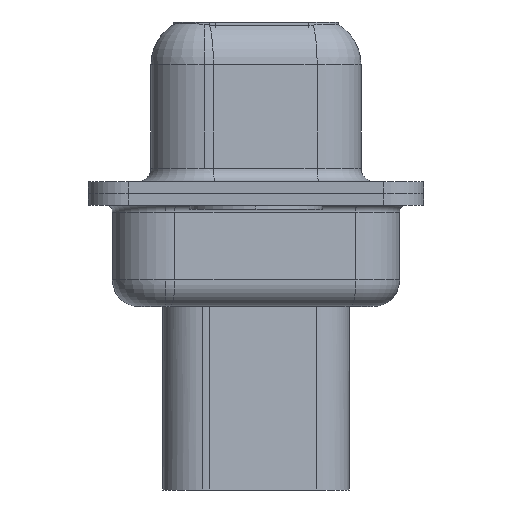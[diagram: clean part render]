
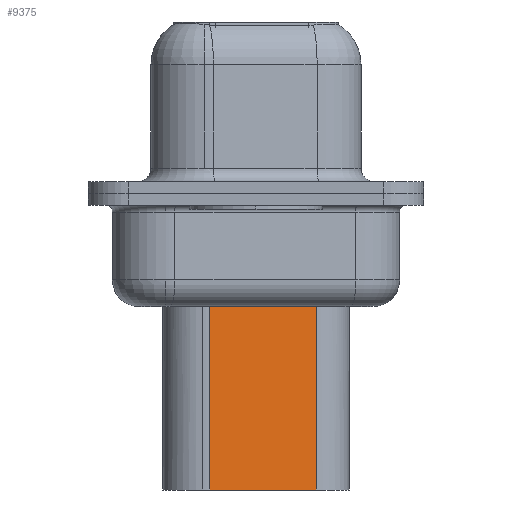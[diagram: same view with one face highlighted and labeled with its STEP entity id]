
A CAD part, left-side view. The second image highlights one B-rep face of the part: STEP entity #9375.
In plain terms, the highlighted planar face has unit normal (-0.985, -0.174, 0).
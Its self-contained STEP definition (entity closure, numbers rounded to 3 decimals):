
#28 = VECTOR ( 'NONE', #10240, 1000. ) ;
#296 = DIRECTION ( 'NONE',  ( -0.174, 0.985, 0. ) ) ;
#1216 = LINE ( 'NONE', #3573, #3936 ) ;
#1511 = EDGE_CURVE ( 'NONE', #6436, #9816, #1216, .T. ) ;
#1523 = EDGE_LOOP ( 'NONE', ( #1975, #10669, #6232, #9168 ) ) ;
#1604 = CARTESIAN_POINT ( 'NONE',  ( 4.524, 1.74, -3.975 ) ) ;
#1975 = ORIENTED_EDGE ( 'NONE', *, *, #5110, .F. ) ;
#2356 = EDGE_CURVE ( 'NONE', #5123, #9816, #5255, .T. ) ;
#3018 = PLANE ( 'NONE',  #7346 ) ;
#3091 = CARTESIAN_POINT ( 'NONE',  ( 5.229, -2.26, -3.975 ) ) ;
#3573 = CARTESIAN_POINT ( 'NONE',  ( 4.524, 1.74, -3.1 ) ) ;
#3772 = CARTESIAN_POINT ( 'NONE',  ( 4.524, 1.74, -3.1 ) ) ;
#3780 = DIRECTION ( 'NONE',  ( 0., 0., -1. ) ) ;
#3936 = VECTOR ( 'NONE', #3780, 1000. ) ;
#3957 = VERTEX_POINT ( 'NONE', #3091 ) ;
#4411 = LINE ( 'NONE', #9379, #4793 ) ;
#4793 = VECTOR ( 'NONE', #10362, 1000. ) ;
#5110 = EDGE_CURVE ( 'NONE', #3957, #5123, #4411, .T. ) ;
#5123 = VERTEX_POINT ( 'NONE', #8883 ) ;
#5255 = LINE ( 'NONE', #5914, #7487 ) ;
#5568 = FACE_OUTER_BOUND ( 'NONE', #1523, .T. ) ;
#5914 = CARTESIAN_POINT ( 'NONE',  ( 4.524, 1.74, -11.15 ) ) ;
#6232 = ORIENTED_EDGE ( 'NONE', *, *, #1511, .T. ) ;
#6352 = DIRECTION ( 'NONE',  ( 0.174, -0.985, 0. ) ) ;
#6436 = VERTEX_POINT ( 'NONE', #1604 ) ;
#7223 = CARTESIAN_POINT ( 'NONE',  ( 4.524, 1.74, -11.15 ) ) ;
#7233 = DIRECTION ( 'NONE',  ( -0.985, -0.174, 0. ) ) ;
#7346 = AXIS2_PLACEMENT_3D ( 'NONE', #3772, #7233, #6352 ) ;
#7487 = VECTOR ( 'NONE', #296, 1000. ) ;
#7738 = LINE ( 'NONE', #9536, #28 ) ;
#8727 = EDGE_CURVE ( 'NONE', #3957, #6436, #7738, .T. ) ;
#8883 = CARTESIAN_POINT ( 'NONE',  ( 5.229, -2.26, -11.15 ) ) ;
#9168 = ORIENTED_EDGE ( 'NONE', *, *, #2356, .F. ) ;
#9375 = ADVANCED_FACE ( 'NONE', ( #5568 ), #3018, .T. ) ;
#9379 = CARTESIAN_POINT ( 'NONE',  ( 5.229, -2.26, -3.1 ) ) ;
#9536 = CARTESIAN_POINT ( 'NONE',  ( 4.353, 2.709, -3.975 ) ) ;
#9816 = VERTEX_POINT ( 'NONE', #7223 ) ;
#10240 = DIRECTION ( 'NONE',  ( -0.174, 0.985, 0. ) ) ;
#10362 = DIRECTION ( 'NONE',  ( 0., 0., -1. ) ) ;
#10669 = ORIENTED_EDGE ( 'NONE', *, *, #8727, .T. ) ;
